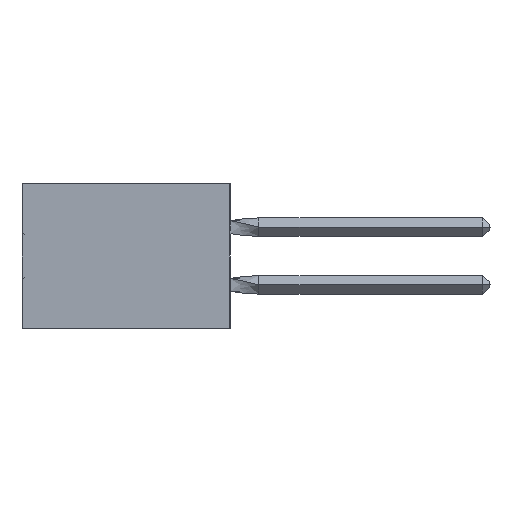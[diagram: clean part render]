
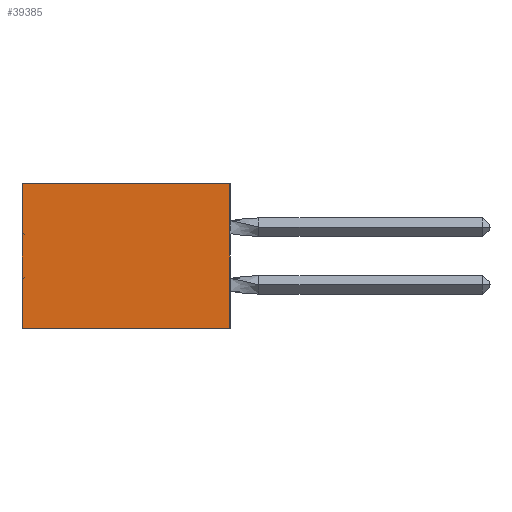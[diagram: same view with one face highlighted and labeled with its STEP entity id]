
A CAD part, left-side view. The second image highlights one B-rep face of the part: STEP entity #39385.
In plain terms, the highlighted planar face has unit normal (-1, 0, 0).
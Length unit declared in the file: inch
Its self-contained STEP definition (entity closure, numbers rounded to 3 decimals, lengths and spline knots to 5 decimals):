
#2138 = EDGE_CURVE ( 'NONE', #12215, #16108, #55888, .T. ) ;
#2240 = CARTESIAN_POINT ( 'NONE',  ( 0.305, 0.72, -0.5 ) ) ;
#3846 = DIRECTION ( 'NONE',  ( 0., 0., -1. ) ) ;
#4848 = VERTEX_POINT ( 'NONE', #17329 ) ;
#8527 = PLANE ( 'NONE',  #28221 ) ;
#8720 = LINE ( 'NONE', #2240, #43674 ) ;
#11097 = ORIENTED_EDGE ( 'NONE', *, *, #30811, .T. ) ;
#12215 = VERTEX_POINT ( 'NONE', #17442 ) ;
#12443 = FACE_OUTER_BOUND ( 'NONE', #43296, .T. ) ;
#12511 = CARTESIAN_POINT ( 'NONE',  ( 0.305, 0., -0.5 ) ) ;
#13418 = CARTESIAN_POINT ( 'NONE',  ( 0.305, 0.72, -0.5 ) ) ;
#16108 = VERTEX_POINT ( 'NONE', #13418 ) ;
#17329 = CARTESIAN_POINT ( 'NONE',  ( 0.305, 0., 0. ) ) ;
#17442 = CARTESIAN_POINT ( 'NONE',  ( 0.305, 0., -0.5 ) ) ;
#17571 = DIRECTION ( 'NONE',  ( 0., 1., 0. ) ) ;
#21356 = CARTESIAN_POINT ( 'NONE',  ( 0.305, 0., -0.5 ) ) ;
#25303 = CARTESIAN_POINT ( 'NONE',  ( 0.305, 0., -0.5 ) ) ;
#25521 = DIRECTION ( 'NONE',  ( 0., 1., 0. ) ) ;
#27990 = LINE ( 'NONE', #25303, #29403 ) ;
#28221 = AXIS2_PLACEMENT_3D ( 'NONE', #21356, #39555, #3846 ) ;
#29207 = DIRECTION ( 'NONE',  ( 0., 0., -1. ) ) ;
#29403 = VECTOR ( 'NONE', #29207, 39.37008 ) ;
#30375 = EDGE_CURVE ( 'NONE', #4848, #39156, #49890, .T. ) ;
#30811 = EDGE_CURVE ( 'NONE', #39156, #16108, #8720, .T. ) ;
#39156 = VERTEX_POINT ( 'NONE', #53739 ) ;
#39385 = ADVANCED_FACE ( 'NONE', ( #12443 ), #8527, .F. ) ;
#39555 = DIRECTION ( 'NONE',  ( 1., 0., 0. ) ) ;
#39839 = CARTESIAN_POINT ( 'NONE',  ( 0.305, 0., 0. ) ) ;
#40120 = ORIENTED_EDGE ( 'NONE', *, *, #2138, .F. ) ;
#42662 = DIRECTION ( 'NONE',  ( 0., 0., -1. ) ) ;
#43296 = EDGE_LOOP ( 'NONE', ( #11097, #40120, #44468, #54734 ) ) ;
#43674 = VECTOR ( 'NONE', #42662, 39.37008 ) ;
#44468 = ORIENTED_EDGE ( 'NONE', *, *, #57246, .F. ) ;
#49890 = LINE ( 'NONE', #39839, #56084 ) ;
#53152 = VECTOR ( 'NONE', #25521, 39.37008 ) ;
#53739 = CARTESIAN_POINT ( 'NONE',  ( 0.305, 0.72, 0. ) ) ;
#54734 = ORIENTED_EDGE ( 'NONE', *, *, #30375, .T. ) ;
#55888 = LINE ( 'NONE', #12511, #53152 ) ;
#56084 = VECTOR ( 'NONE', #17571, 39.37008 ) ;
#57246 = EDGE_CURVE ( 'NONE', #4848, #12215, #27990, .T. ) ;
